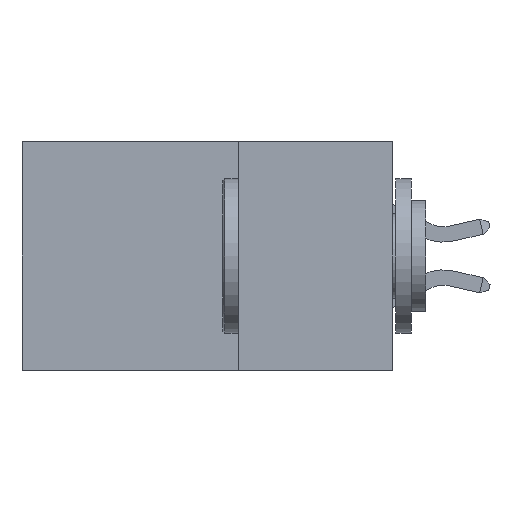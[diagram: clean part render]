
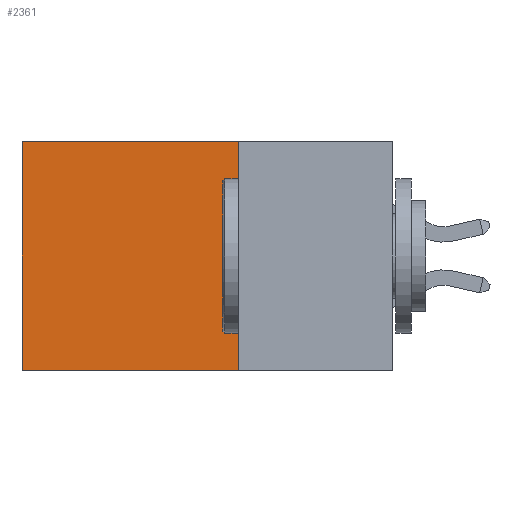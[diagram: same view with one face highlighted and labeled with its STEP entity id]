
A CAD part, left-side view. The second image highlights one B-rep face of the part: STEP entity #2361.
In plain terms, the highlighted planar face has unit normal (-1, 0, 0).
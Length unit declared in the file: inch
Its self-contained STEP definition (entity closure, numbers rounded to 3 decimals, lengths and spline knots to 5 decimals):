
#81 = EDGE_CURVE ( 'NONE', #3953, #6066, #11748, .T. ) ;
#471 = ORIENTED_EDGE ( 'NONE', *, *, #10003, .F. ) ;
#487 = LINE ( 'NONE', #14576, #2078 ) ;
#947 = EDGE_CURVE ( 'NONE', #11196, #9653, #7404, .T. ) ;
#2078 = VECTOR ( 'NONE', #3372, 39.37008 ) ;
#2361 = ADVANCED_FACE ( 'NONE', ( #3039 ), #7772, .F. ) ;
#3039 = FACE_OUTER_BOUND ( 'NONE', #6664, .T. ) ;
#3049 = LINE ( 'NONE', #13353, #13488 ) ;
#3372 = DIRECTION ( 'NONE',  ( 0., 0., -1. ) ) ;
#3953 = VERTEX_POINT ( 'NONE', #4279 ) ;
#3972 = DIRECTION ( 'NONE',  ( 0., 1., 0. ) ) ;
#4279 = CARTESIAN_POINT ( 'NONE',  ( 0.2875, 0.25, -0.37 ) ) ;
#5406 = CARTESIAN_POINT ( 'NONE',  ( 0.2875, 0.6, 0. ) ) ;
#6066 = VERTEX_POINT ( 'NONE', #10167 ) ;
#6357 = AXIS2_PLACEMENT_3D ( 'NONE', #10341, #12616, #8953 ) ;
#6664 = EDGE_LOOP ( 'NONE', ( #15565, #12588, #471, #6883 ) ) ;
#6806 = VECTOR ( 'NONE', #3972, 39.37008 ) ;
#6883 = ORIENTED_EDGE ( 'NONE', *, *, #947, .T. ) ;
#7253 = DIRECTION ( 'NONE',  ( 0., 1., 0. ) ) ;
#7404 = LINE ( 'NONE', #11066, #12338 ) ;
#7772 = PLANE ( 'NONE',  #6357 ) ;
#8953 = DIRECTION ( 'NONE',  ( 0., 0., -1. ) ) ;
#9653 = VERTEX_POINT ( 'NONE', #5406 ) ;
#10003 = EDGE_CURVE ( 'NONE', #11196, #3953, #3049, .T. ) ;
#10167 = CARTESIAN_POINT ( 'NONE',  ( 0.2875, 0.6, -0.37 ) ) ;
#10341 = CARTESIAN_POINT ( 'NONE',  ( 0.2875, 0.25, 0. ) ) ;
#11066 = CARTESIAN_POINT ( 'NONE',  ( 0.2875, 0.25, 0. ) ) ;
#11196 = VERTEX_POINT ( 'NONE', #12678 ) ;
#11748 = LINE ( 'NONE', #12748, #6806 ) ;
#12338 = VECTOR ( 'NONE', #7253, 39.37008 ) ;
#12588 = ORIENTED_EDGE ( 'NONE', *, *, #81, .F. ) ;
#12616 = DIRECTION ( 'NONE',  ( 1., 0., 0. ) ) ;
#12678 = CARTESIAN_POINT ( 'NONE',  ( 0.2875, 0.25, 0. ) ) ;
#12748 = CARTESIAN_POINT ( 'NONE',  ( 0.2875, 0.25, -0.37 ) ) ;
#13353 = CARTESIAN_POINT ( 'NONE',  ( 0.2875, 0.25, 0. ) ) ;
#13413 = DIRECTION ( 'NONE',  ( 0., 0., -1. ) ) ;
#13488 = VECTOR ( 'NONE', #13413, 39.37008 ) ;
#14576 = CARTESIAN_POINT ( 'NONE',  ( 0.2875, 0.6, 0. ) ) ;
#15565 = ORIENTED_EDGE ( 'NONE', *, *, #16196, .T. ) ;
#16196 = EDGE_CURVE ( 'NONE', #9653, #6066, #487, .T. ) ;
